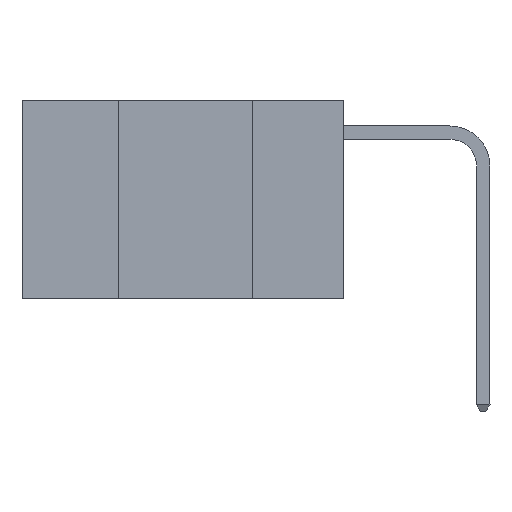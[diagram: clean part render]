
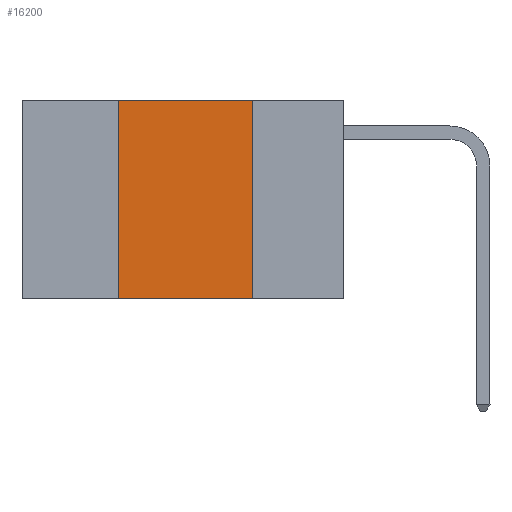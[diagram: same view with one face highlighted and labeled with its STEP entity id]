
A CAD part, left-side view. The second image highlights one B-rep face of the part: STEP entity #16200.
In plain terms, the highlighted planar face has unit normal (-1, 0, 0).
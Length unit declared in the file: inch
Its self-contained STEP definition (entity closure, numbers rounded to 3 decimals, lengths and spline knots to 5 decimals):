
#384 = ORIENTED_EDGE ( 'NONE', *, *, #17652, .F. ) ;
#426 = CARTESIAN_POINT ( 'NONE',  ( 0., 0.17, -0.37 ) ) ;
#1466 = VECTOR ( 'NONE', #15094, 39.37008 ) ;
#1677 = ORIENTED_EDGE ( 'NONE', *, *, #5909, .F. ) ;
#2329 = PLANE ( 'NONE',  #15083 ) ;
#2892 = ORIENTED_EDGE ( 'NONE', *, *, #12911, .T. ) ;
#3847 = ORIENTED_EDGE ( 'NONE', *, *, #18848, .F. ) ;
#3986 = CARTESIAN_POINT ( 'NONE',  ( 0., 0.42, 0. ) ) ;
#4141 = CARTESIAN_POINT ( 'NONE',  ( 0., 0.6, 0. ) ) ;
#4482 = VECTOR ( 'NONE', #9148, 39.37008 ) ;
#5890 = DIRECTION ( 'NONE',  ( 1., 0., 0. ) ) ;
#5909 = EDGE_CURVE ( 'NONE', #11668, #17693, #6212, .T. ) ;
#6212 = LINE ( 'NONE', #22065, #1466 ) ;
#6637 = CARTESIAN_POINT ( 'NONE',  ( 0., 0.42, 0. ) ) ;
#6707 = DIRECTION ( 'NONE',  ( 0., 0., 1. ) ) ;
#7324 = CARTESIAN_POINT ( 'NONE',  ( 0., 0.17, 0. ) ) ;
#7426 = DIRECTION ( 'NONE',  ( 0., -1., 0. ) ) ;
#7581 = VECTOR ( 'NONE', #6707, 39.37008 ) ;
#7812 = LINE ( 'NONE', #14464, #12036 ) ;
#8135 = LINE ( 'NONE', #6637, #7581 ) ;
#9148 = DIRECTION ( 'NONE',  ( 0., 0., -1. ) ) ;
#11668 = VERTEX_POINT ( 'NONE', #3986 ) ;
#12036 = VECTOR ( 'NONE', #7426, 39.37008 ) ;
#12194 = CARTESIAN_POINT ( 'NONE',  ( 0., 0.17, 0. ) ) ;
#12493 = EDGE_LOOP ( 'NONE', ( #3847, #1677, #384, #2892 ) ) ;
#12911 = EDGE_CURVE ( 'NONE', #14851, #17274, #7812, .T. ) ;
#13180 = FACE_OUTER_BOUND ( 'NONE', #12493, .T. ) ;
#14464 = CARTESIAN_POINT ( 'NONE',  ( 0., 0.6, -0.37 ) ) ;
#14851 = VERTEX_POINT ( 'NONE', #16606 ) ;
#15083 = AXIS2_PLACEMENT_3D ( 'NONE', #4141, #5890, #18311 ) ;
#15094 = DIRECTION ( 'NONE',  ( 0., -1., 0. ) ) ;
#16200 = ADVANCED_FACE ( 'NONE', ( #13180 ), #2329, .F. ) ;
#16606 = CARTESIAN_POINT ( 'NONE',  ( 0., 0.42, -0.37 ) ) ;
#17274 = VERTEX_POINT ( 'NONE', #426 ) ;
#17652 = EDGE_CURVE ( 'NONE', #14851, #11668, #8135, .T. ) ;
#17693 = VERTEX_POINT ( 'NONE', #12194 ) ;
#18311 = DIRECTION ( 'NONE',  ( 0., 0., -1. ) ) ;
#18848 = EDGE_CURVE ( 'NONE', #17693, #17274, #19185, .T. ) ;
#19185 = LINE ( 'NONE', #7324, #4482 ) ;
#22065 = CARTESIAN_POINT ( 'NONE',  ( 0., 0.6, 0. ) ) ;
